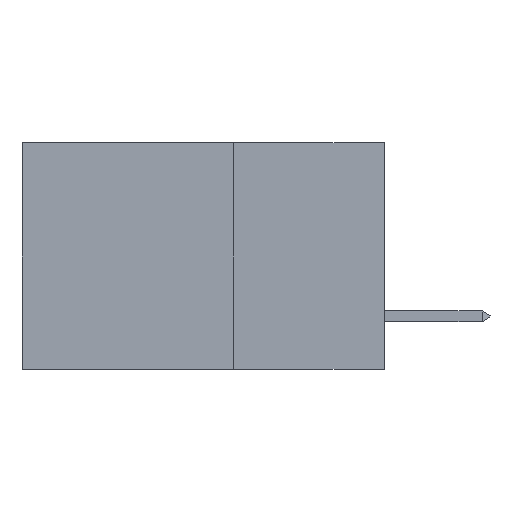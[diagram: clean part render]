
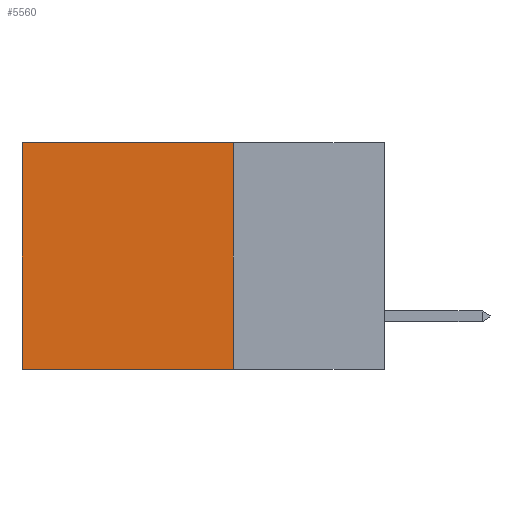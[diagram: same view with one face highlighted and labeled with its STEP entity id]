
A CAD part, left-side view. The second image highlights one B-rep face of the part: STEP entity #5560.
In plain terms, the highlighted planar face has unit normal (-1, 0, 0).
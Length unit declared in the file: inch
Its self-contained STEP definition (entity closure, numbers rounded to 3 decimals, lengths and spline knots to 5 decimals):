
#130 = CARTESIAN_POINT ( 'NONE',  ( 0.2875, 0.25, -0.375 ) ) ;
#1488 = VECTOR ( 'NONE', #13220, 39.37008 ) ;
#2067 = VERTEX_POINT ( 'NONE', #9728 ) ;
#2739 = DIRECTION ( 'NONE',  ( 0., 1., 0. ) ) ;
#2787 = CARTESIAN_POINT ( 'NONE',  ( 0.2875, 0.25, -0.375 ) ) ;
#4110 = DIRECTION ( 'NONE',  ( 0., 0., -1. ) ) ;
#4244 = ORIENTED_EDGE ( 'NONE', *, *, #8677, .T. ) ;
#4411 = EDGE_LOOP ( 'NONE', ( #9919, #15623, #14943, #4244 ) ) ;
#5008 = AXIS2_PLACEMENT_3D ( 'NONE', #130, #14078, #15533 ) ;
#5179 = LINE ( 'NONE', #16023, #1488 ) ;
#5560 = ADVANCED_FACE ( 'NONE', ( #14900 ), #14137, .F. ) ;
#7302 = DIRECTION ( 'NONE',  ( 0., 1., 0. ) ) ;
#8088 = CARTESIAN_POINT ( 'NONE',  ( 0.2875, 0.25, -0.375 ) ) ;
#8677 = EDGE_CURVE ( 'NONE', #15610, #2067, #14330, .T. ) ;
#8839 = CARTESIAN_POINT ( 'NONE',  ( 0.2875, 0.25, 0. ) ) ;
#9728 = CARTESIAN_POINT ( 'NONE',  ( 0.2875, 0.6, 0. ) ) ;
#9919 = ORIENTED_EDGE ( 'NONE', *, *, #13093, .T. ) ;
#10611 = VECTOR ( 'NONE', #2739, 39.37008 ) ;
#11961 = CARTESIAN_POINT ( 'NONE',  ( 0.2875, 0.6, -0.375 ) ) ;
#12415 = LINE ( 'NONE', #16815, #17034 ) ;
#13093 = EDGE_CURVE ( 'NONE', #2067, #17996, #5179, .T. ) ;
#13220 = DIRECTION ( 'NONE',  ( 0., 0., -1. ) ) ;
#13389 = EDGE_CURVE ( 'NONE', #15610, #16603, #15561, .T. ) ;
#14078 = DIRECTION ( 'NONE',  ( 1., 0., 0. ) ) ;
#14137 = PLANE ( 'NONE',  #5008 ) ;
#14330 = LINE ( 'NONE', #17928, #10611 ) ;
#14900 = FACE_OUTER_BOUND ( 'NONE', #4411, .T. ) ;
#14943 = ORIENTED_EDGE ( 'NONE', *, *, #13389, .F. ) ;
#15405 = EDGE_CURVE ( 'NONE', #16603, #17996, #12415, .T. ) ;
#15533 = DIRECTION ( 'NONE',  ( 0., 0., -1. ) ) ;
#15561 = LINE ( 'NONE', #8088, #17723 ) ;
#15610 = VERTEX_POINT ( 'NONE', #8839 ) ;
#15623 = ORIENTED_EDGE ( 'NONE', *, *, #15405, .F. ) ;
#16023 = CARTESIAN_POINT ( 'NONE',  ( 0.2875, 0.6, -0.375 ) ) ;
#16603 = VERTEX_POINT ( 'NONE', #2787 ) ;
#16815 = CARTESIAN_POINT ( 'NONE',  ( 0.2875, 0.25, -0.375 ) ) ;
#17034 = VECTOR ( 'NONE', #7302, 39.37008 ) ;
#17723 = VECTOR ( 'NONE', #4110, 39.37008 ) ;
#17928 = CARTESIAN_POINT ( 'NONE',  ( 0.2875, 0.25, 0. ) ) ;
#17996 = VERTEX_POINT ( 'NONE', #11961 ) ;
